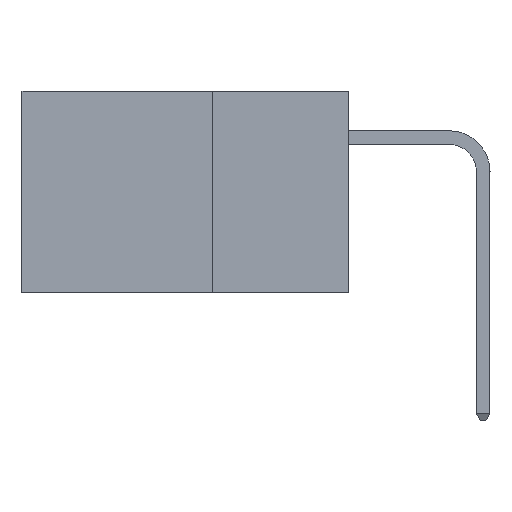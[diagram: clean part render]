
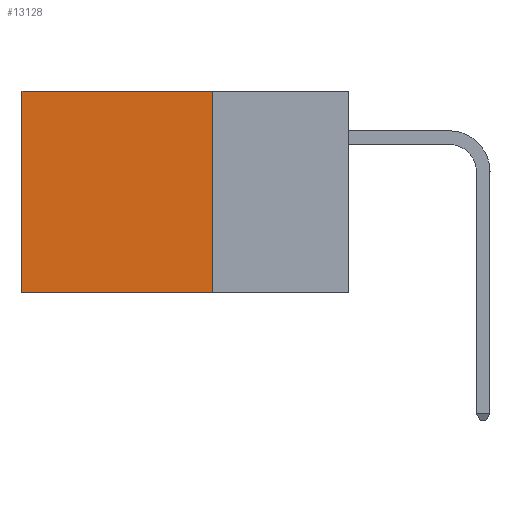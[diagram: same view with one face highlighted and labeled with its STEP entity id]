
A CAD part, left-side view. The second image highlights one B-rep face of the part: STEP entity #13128.
In plain terms, the highlighted planar face has unit normal (-1, 0, 0).
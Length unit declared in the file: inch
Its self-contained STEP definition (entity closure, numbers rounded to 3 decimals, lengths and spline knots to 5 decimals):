
#297 = CARTESIAN_POINT ( 'NONE',  ( 0.2875, 0.25, -0.37 ) ) ;
#814 = CARTESIAN_POINT ( 'NONE',  ( 0.2875, 0.6, -0.37 ) ) ;
#1444 = VERTEX_POINT ( 'NONE', #814 ) ;
#1552 = VECTOR ( 'NONE', #13254, 39.37008 ) ;
#1928 = DIRECTION ( 'NONE',  ( 0., 1., 0. ) ) ;
#2393 = CARTESIAN_POINT ( 'NONE',  ( 0.2875, 0.6, 0. ) ) ;
#2906 = LINE ( 'NONE', #297, #6211 ) ;
#3365 = CARTESIAN_POINT ( 'NONE',  ( 0.2875, 0.25, 0. ) ) ;
#3766 = DIRECTION ( 'NONE',  ( 0., 1., 0. ) ) ;
#4153 = ORIENTED_EDGE ( 'NONE', *, *, #7112, .T. ) ;
#4311 = ORIENTED_EDGE ( 'NONE', *, *, #20052, .T. ) ;
#4664 = LINE ( 'NONE', #3365, #16848 ) ;
#5512 = AXIS2_PLACEMENT_3D ( 'NONE', #6047, #17120, #7675 ) ;
#5877 = LINE ( 'NONE', #10694, #1552 ) ;
#6047 = CARTESIAN_POINT ( 'NONE',  ( 0.2875, 0.25, 0. ) ) ;
#6211 = VECTOR ( 'NONE', #1928, 39.37008 ) ;
#6587 = VECTOR ( 'NONE', #3766, 39.37008 ) ;
#7049 = CARTESIAN_POINT ( 'NONE',  ( 0.2875, 0.25, 0. ) ) ;
#7112 = EDGE_CURVE ( 'NONE', #8237, #7704, #10883, .T. ) ;
#7675 = DIRECTION ( 'NONE',  ( 0., 0., -1. ) ) ;
#7704 = VERTEX_POINT ( 'NONE', #2393 ) ;
#8237 = VERTEX_POINT ( 'NONE', #7049 ) ;
#8253 = DIRECTION ( 'NONE',  ( 0., 0., -1. ) ) ;
#8587 = CARTESIAN_POINT ( 'NONE',  ( 0.2875, 0.25, 0. ) ) ;
#8851 = VERTEX_POINT ( 'NONE', #19754 ) ;
#10694 = CARTESIAN_POINT ( 'NONE',  ( 0.2875, 0.6, 0. ) ) ;
#10883 = LINE ( 'NONE', #8587, #6587 ) ;
#11148 = EDGE_CURVE ( 'NONE', #8851, #1444, #2906, .T. ) ;
#12135 = EDGE_CURVE ( 'NONE', #8237, #8851, #4664, .T. ) ;
#13128 = ADVANCED_FACE ( 'NONE', ( #15354 ), #15576, .F. ) ;
#13254 = DIRECTION ( 'NONE',  ( 0., 0., -1. ) ) ;
#15354 = FACE_OUTER_BOUND ( 'NONE', #16174, .T. ) ;
#15576 = PLANE ( 'NONE',  #5512 ) ;
#16174 = EDGE_LOOP ( 'NONE', ( #4311, #16817, #16193, #4153 ) ) ;
#16193 = ORIENTED_EDGE ( 'NONE', *, *, #12135, .F. ) ;
#16817 = ORIENTED_EDGE ( 'NONE', *, *, #11148, .F. ) ;
#16848 = VECTOR ( 'NONE', #8253, 39.37008 ) ;
#17120 = DIRECTION ( 'NONE',  ( 1., 0., 0. ) ) ;
#19754 = CARTESIAN_POINT ( 'NONE',  ( 0.2875, 0.25, -0.37 ) ) ;
#20052 = EDGE_CURVE ( 'NONE', #7704, #1444, #5877, .T. ) ;
